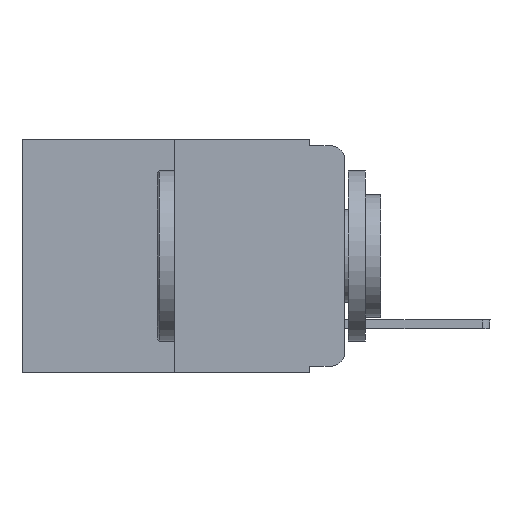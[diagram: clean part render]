
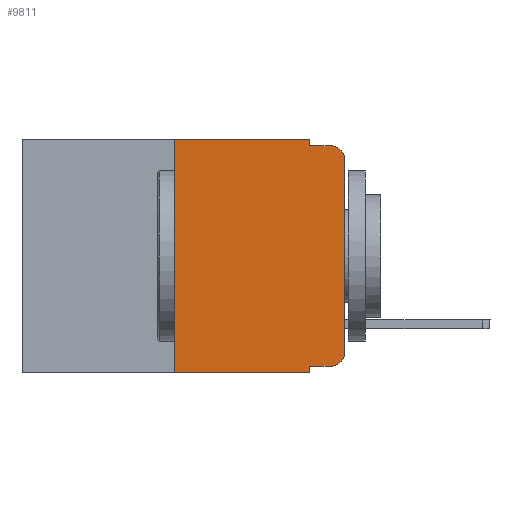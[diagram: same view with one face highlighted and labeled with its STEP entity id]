
A CAD part, left-side view. The second image highlights one B-rep face of the part: STEP entity #9811.
In plain terms, the highlighted planar face has unit normal (-1, 0, 0).
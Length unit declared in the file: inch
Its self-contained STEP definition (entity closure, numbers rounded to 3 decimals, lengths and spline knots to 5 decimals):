
#111 = ORIENTED_EDGE ( 'NONE', *, *, #161, .F. ) ;
#161 = EDGE_CURVE ( 'NONE', #3372, #4163, #869, .T. ) ;
#319 = CIRCLE ( 'NONE', #5641, 0.02 ) ;
#344 = VERTEX_POINT ( 'NONE', #11389 ) ;
#355 = EDGE_CURVE ( 'NONE', #10958, #4721, #14828, .T. ) ;
#869 = LINE ( 'NONE', #14677, #11682 ) ;
#1631 = VECTOR ( 'NONE', #8828, 39.37008 ) ;
#1685 = DIRECTION ( 'NONE',  ( 0., 0., -1. ) ) ;
#1724 = DIRECTION ( 'NONE',  ( 0., 0., -1. ) ) ;
#2103 = CARTESIAN_POINT ( 'NONE',  ( 0., 0., 0. ) ) ;
#2225 = EDGE_CURVE ( 'NONE', #14433, #10958, #2321, .T. ) ;
#2279 = ORIENTED_EDGE ( 'NONE', *, *, #355, .F. ) ;
#2321 = LINE ( 'NONE', #7845, #5346 ) ;
#2769 = EDGE_CURVE ( 'NONE', #3970, #4599, #9477, .T. ) ;
#3010 = EDGE_CURVE ( 'NONE', #14433, #6824, #14505, .T. ) ;
#3254 = LINE ( 'NONE', #2103, #1631 ) ;
#3372 = VERTEX_POINT ( 'NONE', #9825 ) ;
#3612 = AXIS2_PLACEMENT_3D ( 'NONE', #8734, #6403, #1724 ) ;
#3970 = VERTEX_POINT ( 'NONE', #10095 ) ;
#4163 = VERTEX_POINT ( 'NONE', #10694 ) ;
#4564 = ORIENTED_EDGE ( 'NONE', *, *, #6588, .T. ) ;
#4592 = CARTESIAN_POINT ( 'NONE',  ( 0., 0.051, 0. ) ) ;
#4599 = VERTEX_POINT ( 'NONE', #12898 ) ;
#4721 = VERTEX_POINT ( 'NONE', #4843 ) ;
#4843 = CARTESIAN_POINT ( 'NONE',  ( 0., 0.051, 0. ) ) ;
#4915 = VECTOR ( 'NONE', #12293, 39.37008 ) ;
#5043 = EDGE_CURVE ( 'NONE', #344, #8969, #3254, .T. ) ;
#5103 = CARTESIAN_POINT ( 'NONE',  ( 0., 0.25, -0.343 ) ) ;
#5346 = VECTOR ( 'NONE', #8062, 39.37008 ) ;
#5641 = AXIS2_PLACEMENT_3D ( 'NONE', #5944, #12641, #7087 ) ;
#5924 = CARTESIAN_POINT ( 'NONE',  ( 0., 0.051, -0.343 ) ) ;
#5944 = CARTESIAN_POINT ( 'NONE',  ( 0., 0.02, -0.313 ) ) ;
#6403 = DIRECTION ( 'NONE',  ( -1., 0., 0. ) ) ;
#6588 = EDGE_CURVE ( 'NONE', #8969, #4163, #10841, .T. ) ;
#6824 = VERTEX_POINT ( 'NONE', #5924 ) ;
#6915 = DIRECTION ( 'NONE',  ( 0., -1., 0. ) ) ;
#7087 = DIRECTION ( 'NONE',  ( 0., 0., -1. ) ) ;
#7845 = CARTESIAN_POINT ( 'NONE',  ( 0., 0.25, 0. ) ) ;
#8062 = DIRECTION ( 'NONE',  ( 0., 0., 1. ) ) ;
#8114 = CARTESIAN_POINT ( 'NONE',  ( 0., 0.051, -0.333 ) ) ;
#8254 = CARTESIAN_POINT ( 'NONE',  ( 0., 0.473, 0. ) ) ;
#8579 = DIRECTION ( 'NONE',  ( 0., -1., 0. ) ) ;
#8734 = CARTESIAN_POINT ( 'NONE',  ( 0., 0.02, -0.03 ) ) ;
#8828 = DIRECTION ( 'NONE',  ( 0., 0., 1. ) ) ;
#8969 = VERTEX_POINT ( 'NONE', #9655 ) ;
#9193 = LINE ( 'NONE', #4592, #10457 ) ;
#9357 = VECTOR ( 'NONE', #10691, 39.37008 ) ;
#9453 = ORIENTED_EDGE ( 'NONE', *, *, #2225, .F. ) ;
#9477 = LINE ( 'NONE', #8114, #9357 ) ;
#9655 = CARTESIAN_POINT ( 'NONE',  ( 0., 0., -0.03 ) ) ;
#9691 = PLANE ( 'NONE',  #11611 ) ;
#9811 = ADVANCED_FACE ( 'NONE', ( #12064 ), #9691, .F. ) ;
#9825 = CARTESIAN_POINT ( 'NONE',  ( 0., 0.051, -0.01 ) ) ;
#9976 = VECTOR ( 'NONE', #6915, 39.37008 ) ;
#10095 = CARTESIAN_POINT ( 'NONE',  ( 0., 0.051, -0.333 ) ) ;
#10127 = LINE ( 'NONE', #12229, #4915 ) ;
#10214 = VECTOR ( 'NONE', #10844, 39.37008 ) ;
#10289 = ORIENTED_EDGE ( 'NONE', *, *, #13831, .F. ) ;
#10457 = VECTOR ( 'NONE', #11405, 39.37008 ) ;
#10691 = DIRECTION ( 'NONE',  ( 0., -1., 0. ) ) ;
#10694 = CARTESIAN_POINT ( 'NONE',  ( 0., 0.02, -0.01 ) ) ;
#10841 = CIRCLE ( 'NONE', #3612, 0.02 ) ;
#10844 = DIRECTION ( 'NONE',  ( 0., -1., 0. ) ) ;
#10958 = VERTEX_POINT ( 'NONE', #12908 ) ;
#11270 = ORIENTED_EDGE ( 'NONE', *, *, #12376, .F. ) ;
#11389 = CARTESIAN_POINT ( 'NONE',  ( 0., 0., -0.313 ) ) ;
#11405 = DIRECTION ( 'NONE',  ( 0., 0., -1. ) ) ;
#11611 = AXIS2_PLACEMENT_3D ( 'NONE', #8254, #14351, #1685 ) ;
#11682 = VECTOR ( 'NONE', #8579, 39.37008 ) ;
#11747 = ORIENTED_EDGE ( 'NONE', *, *, #5043, .T. ) ;
#11826 = ORIENTED_EDGE ( 'NONE', *, *, #12786, .T. ) ;
#12064 = FACE_OUTER_BOUND ( 'NONE', #14475, .T. ) ;
#12229 = CARTESIAN_POINT ( 'NONE',  ( 0., 0.051, 0. ) ) ;
#12293 = DIRECTION ( 'NONE',  ( 0., 0., -1. ) ) ;
#12376 = EDGE_CURVE ( 'NONE', #4721, #3372, #10127, .T. ) ;
#12641 = DIRECTION ( 'NONE',  ( -1., 0., 0. ) ) ;
#12686 = ORIENTED_EDGE ( 'NONE', *, *, #2769, .T. ) ;
#12786 = EDGE_CURVE ( 'NONE', #4599, #344, #319, .T. ) ;
#12898 = CARTESIAN_POINT ( 'NONE',  ( 0., 0.02, -0.333 ) ) ;
#12908 = CARTESIAN_POINT ( 'NONE',  ( 0., 0.25, 0. ) ) ;
#13831 = EDGE_CURVE ( 'NONE', #3970, #6824, #9193, .T. ) ;
#13925 = CARTESIAN_POINT ( 'NONE',  ( 0., 0.473, 0. ) ) ;
#14351 = DIRECTION ( 'NONE',  ( 1., 0., 0. ) ) ;
#14417 = ORIENTED_EDGE ( 'NONE', *, *, #3010, .T. ) ;
#14433 = VERTEX_POINT ( 'NONE', #5103 ) ;
#14434 = CARTESIAN_POINT ( 'NONE',  ( 0., 0.473, -0.343 ) ) ;
#14475 = EDGE_LOOP ( 'NONE', ( #11747, #4564, #111, #11270, #2279, #9453, #14417, #10289, #12686, #11826 ) ) ;
#14505 = LINE ( 'NONE', #14434, #10214 ) ;
#14677 = CARTESIAN_POINT ( 'NONE',  ( 0., 0.051, -0.01 ) ) ;
#14828 = LINE ( 'NONE', #13925, #9976 ) ;
